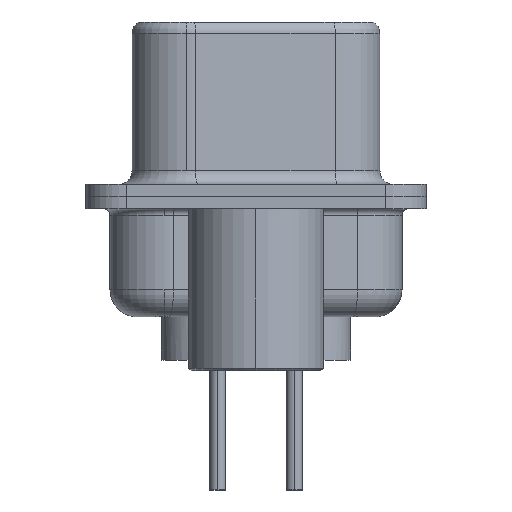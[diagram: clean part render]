
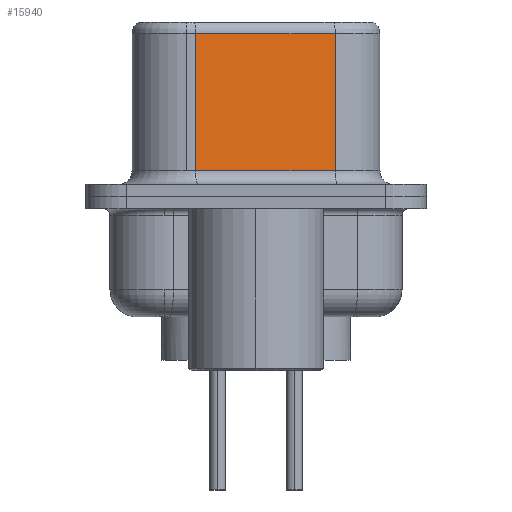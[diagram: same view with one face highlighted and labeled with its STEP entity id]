
A CAD part, left-side view. The second image highlights one B-rep face of the part: STEP entity #15940.
In plain terms, the highlighted planar face has unit normal (-0.985, -0.174, 0).
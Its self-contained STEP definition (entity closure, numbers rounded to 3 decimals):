
#547 = ORIENTED_EDGE ( 'NONE', *, *, #3882, .T. ) ;
#594 = DIRECTION ( 'NONE',  ( 0., 0., -1. ) ) ;
#702 = CARTESIAN_POINT ( 'NONE',  ( 3.665, 2.233, 0.95 ) ) ;
#1735 = EDGE_CURVE ( 'NONE', #21135, #17035, #5579, .T. ) ;
#1812 = CARTESIAN_POINT ( 'NONE',  ( 4.575, -2.927, 0.95 ) ) ;
#1858 = EDGE_CURVE ( 'NONE', #12492, #8480, #16345, .T. ) ;
#3079 = CARTESIAN_POINT ( 'NONE',  ( 4.575, -2.927, 6.02 ) ) ;
#3248 = PLANE ( 'NONE',  #8196 ) ;
#3882 = EDGE_CURVE ( 'NONE', #12492, #21135, #10086, .T. ) ;
#4793 = DIRECTION ( 'NONE',  ( 0.985, 0.174, 0. ) ) ;
#5579 = LINE ( 'NONE', #10710, #5850 ) ;
#5850 = VECTOR ( 'NONE', #594, 1000. ) ;
#7042 = ORIENTED_EDGE ( 'NONE', *, *, #1858, .F. ) ;
#8051 = CARTESIAN_POINT ( 'NONE',  ( 4.575, -2.927, 6.52 ) ) ;
#8196 = AXIS2_PLACEMENT_3D ( 'NONE', #20017, #4793, #11580 ) ;
#8480 = VERTEX_POINT ( 'NONE', #1812 ) ;
#8682 = DIRECTION ( 'NONE',  ( 0.174, -0.985, 0. ) ) ;
#10086 = LINE ( 'NONE', #3079, #19779 ) ;
#10339 = CARTESIAN_POINT ( 'NONE',  ( 4.575, -2.927, 6.02 ) ) ;
#10710 = CARTESIAN_POINT ( 'NONE',  ( 3.665, 2.233, 6.52 ) ) ;
#11580 = DIRECTION ( 'NONE',  ( -0.174, 0.985, 0. ) ) ;
#12492 = VERTEX_POINT ( 'NONE', #10339 ) ;
#12769 = EDGE_LOOP ( 'NONE', ( #7042, #547, #21048, #19667 ) ) ;
#13149 = DIRECTION ( 'NONE',  ( 0., 0., -1. ) ) ;
#13766 = CARTESIAN_POINT ( 'NONE',  ( 4.575, -2.927, 0.95 ) ) ;
#13772 = EDGE_CURVE ( 'NONE', #17035, #8480, #15733, .T. ) ;
#14703 = CARTESIAN_POINT ( 'NONE',  ( 3.665, 2.233, 6.02 ) ) ;
#15733 = LINE ( 'NONE', #13766, #19488 ) ;
#15940 = ADVANCED_FACE ( 'NONE', ( #16872 ), #3248, .F. ) ;
#16345 = LINE ( 'NONE', #8051, #21436 ) ;
#16872 = FACE_OUTER_BOUND ( 'NONE', #12769, .T. ) ;
#17035 = VERTEX_POINT ( 'NONE', #702 ) ;
#19488 = VECTOR ( 'NONE', #8682, 1000. ) ;
#19667 = ORIENTED_EDGE ( 'NONE', *, *, #13772, .T. ) ;
#19779 = VECTOR ( 'NONE', #19850, 1000. ) ;
#19850 = DIRECTION ( 'NONE',  ( -0.174, 0.985, 0. ) ) ;
#20017 = CARTESIAN_POINT ( 'NONE',  ( 4.575, -2.927, 6.52 ) ) ;
#21048 = ORIENTED_EDGE ( 'NONE', *, *, #1735, .T. ) ;
#21135 = VERTEX_POINT ( 'NONE', #14703 ) ;
#21436 = VECTOR ( 'NONE', #13149, 1000. ) ;
